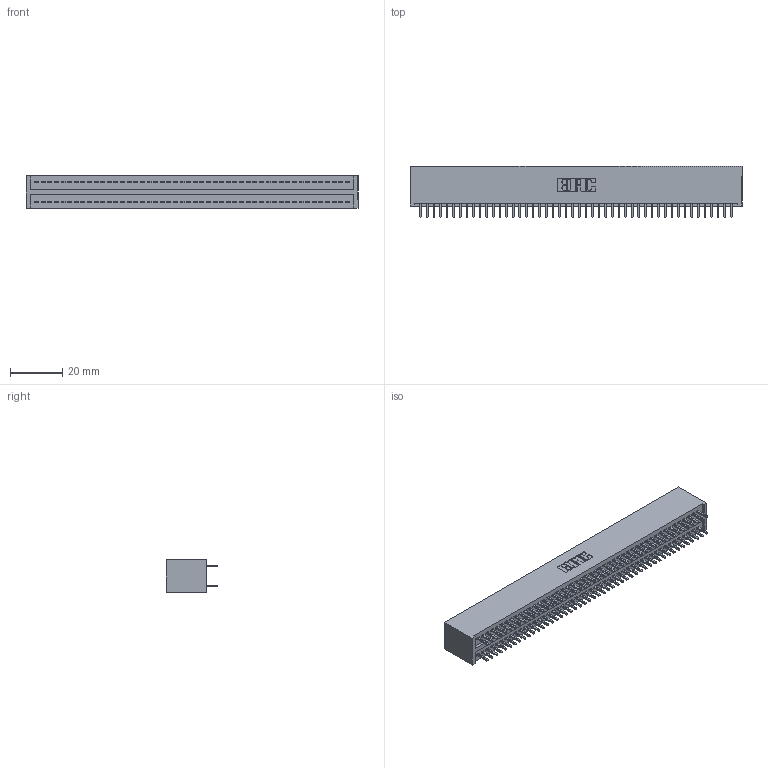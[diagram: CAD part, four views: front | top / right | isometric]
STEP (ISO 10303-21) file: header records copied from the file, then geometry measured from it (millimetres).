
FILE_DESCRIPTION (( 'STEP AP203' ), '1' );
FILE_NAME ('325-096-520-201.STEP', '2020-02-25T06:12:24', ( '' ), ( '' ), 'SwSTEP 2.0', 'SolidWorks 2016', '' );
FILE_SCHEMA (( 'CONFIG_CONTROL_DESIGN' ));
Length unit declared in the file: inch
Products named in the file (3): 325-292-001_325-293-120; 325-096-520-201; 325 Part_Lugless
Assembly tree (97 placements, depth 2):
  325-096-520-201
    325 Part_Lugless
    325-292-001_325-293-120  x96
Bounding box: 127.56 x 19.68 x 12.45 mm (x, y, z)
Volume: 17112.9 mm3; surface area: 21322.2 mm2
Topology: 97 solids, 97 shells, 5098 faces, 15167 edges, 9982 vertices
Faces by surface type: plane 3522, cylinder 1576
Entity records: 29845 total; most frequent: CARTESIAN_POINT 4938, ORIENTED_EDGE 4874, DIRECTION 4201, EDGE_CURVE 2437, LINE 2317, VECTOR 2317, VERTEX_POINT 1622, AXIS2_PLACEMENT_3D 942
